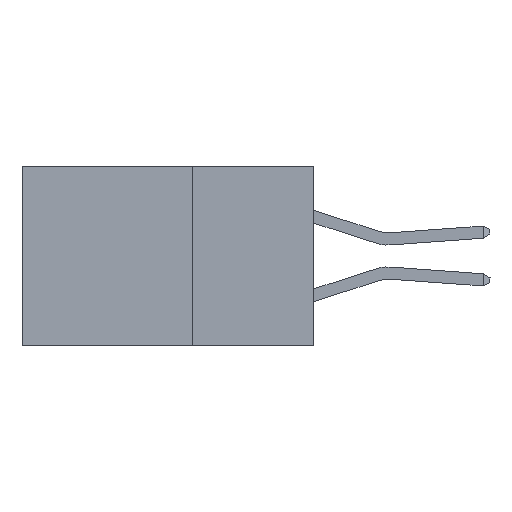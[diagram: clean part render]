
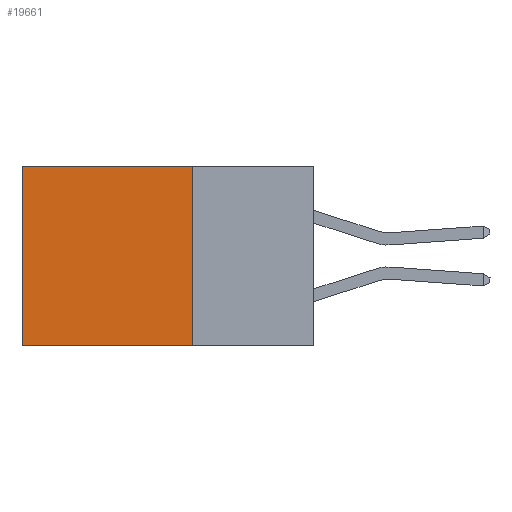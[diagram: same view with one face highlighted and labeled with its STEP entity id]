
A CAD part, left-side view. The second image highlights one B-rep face of the part: STEP entity #19661.
In plain terms, the highlighted planar face has unit normal (-1, 0, 0).
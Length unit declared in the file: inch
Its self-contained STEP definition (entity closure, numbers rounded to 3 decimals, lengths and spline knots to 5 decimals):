
#1543 = CARTESIAN_POINT ( 'NONE',  ( 0.2875, 0.25, 0. ) ) ;
#1744 = CARTESIAN_POINT ( 'NONE',  ( 0.2875, 0.25, 0. ) ) ;
#2245 = ORIENTED_EDGE ( 'NONE', *, *, #17176, .T. ) ;
#2427 = EDGE_CURVE ( 'NONE', #10090, #9321, #9901, .T. ) ;
#3824 = CARTESIAN_POINT ( 'NONE',  ( 0.2875, 0.6, -0.37 ) ) ;
#3898 = VECTOR ( 'NONE', #6891, 39.37008 ) ;
#4103 = CARTESIAN_POINT ( 'NONE',  ( 0.2875, 0.6, 0. ) ) ;
#5306 = DIRECTION ( 'NONE',  ( 1., 0., 0. ) ) ;
#5739 = ORIENTED_EDGE ( 'NONE', *, *, #2427, .T. ) ;
#6222 = EDGE_LOOP ( 'NONE', ( #5739, #21429, #17468, #2245 ) ) ;
#6891 = DIRECTION ( 'NONE',  ( 0., 0., -1. ) ) ;
#7389 = VERTEX_POINT ( 'NONE', #1543 ) ;
#7987 = EDGE_CURVE ( 'NONE', #7389, #12181, #8613, .T. ) ;
#8613 = LINE ( 'NONE', #14004, #3898 ) ;
#9321 = VERTEX_POINT ( 'NONE', #3824 ) ;
#9690 = CARTESIAN_POINT ( 'NONE',  ( 0.2875, 0.25, -0.37 ) ) ;
#9804 = LINE ( 'NONE', #1744, #18193 ) ;
#9901 = LINE ( 'NONE', #11281, #13581 ) ;
#10090 = VERTEX_POINT ( 'NONE', #4103 ) ;
#10805 = FACE_OUTER_BOUND ( 'NONE', #6222, .T. ) ;
#11281 = CARTESIAN_POINT ( 'NONE',  ( 0.2875, 0.6, 0. ) ) ;
#12181 = VERTEX_POINT ( 'NONE', #9690 ) ;
#12307 = LINE ( 'NONE', #20543, #16484 ) ;
#12347 = CARTESIAN_POINT ( 'NONE',  ( 0.2875, 0.25, 0. ) ) ;
#13581 = VECTOR ( 'NONE', #21933, 39.37008 ) ;
#14004 = CARTESIAN_POINT ( 'NONE',  ( 0.2875, 0.25, 0. ) ) ;
#16185 = AXIS2_PLACEMENT_3D ( 'NONE', #12347, #5306, #17780 ) ;
#16484 = VECTOR ( 'NONE', #22412, 39.37008 ) ;
#17176 = EDGE_CURVE ( 'NONE', #7389, #10090, #9804, .T. ) ;
#17468 = ORIENTED_EDGE ( 'NONE', *, *, #7987, .F. ) ;
#17780 = DIRECTION ( 'NONE',  ( 0., 0., -1. ) ) ;
#17804 = DIRECTION ( 'NONE',  ( 0., 1., 0. ) ) ;
#18100 = EDGE_CURVE ( 'NONE', #12181, #9321, #12307, .T. ) ;
#18193 = VECTOR ( 'NONE', #17804, 39.37008 ) ;
#19661 = ADVANCED_FACE ( 'NONE', ( #10805 ), #23040, .F. ) ;
#20543 = CARTESIAN_POINT ( 'NONE',  ( 0.2875, 0.25, -0.37 ) ) ;
#21429 = ORIENTED_EDGE ( 'NONE', *, *, #18100, .F. ) ;
#21933 = DIRECTION ( 'NONE',  ( 0., 0., -1. ) ) ;
#22412 = DIRECTION ( 'NONE',  ( 0., 1., 0. ) ) ;
#23040 = PLANE ( 'NONE',  #16185 ) ;
